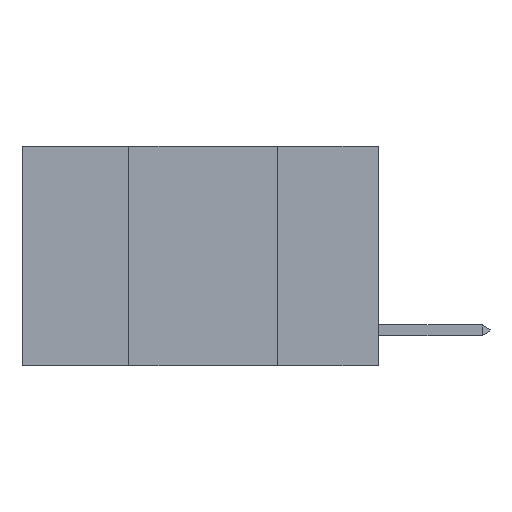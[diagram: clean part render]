
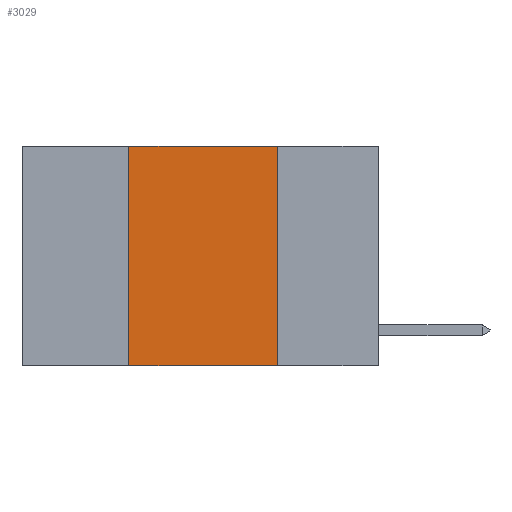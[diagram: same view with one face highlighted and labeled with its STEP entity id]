
A CAD part, left-side view. The second image highlights one B-rep face of the part: STEP entity #3029.
In plain terms, the highlighted planar face has unit normal (-1, 0, 0).
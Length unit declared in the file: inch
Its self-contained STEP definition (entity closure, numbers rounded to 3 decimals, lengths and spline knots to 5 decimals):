
#26 = LINE ( 'NONE', #12752, #2441 ) ;
#378 = EDGE_LOOP ( 'NONE', ( #12110, #11061, #12465, #7243 ) ) ;
#588 = VERTEX_POINT ( 'NONE', #13567 ) ;
#747 = EDGE_CURVE ( 'NONE', #1272, #11423, #3731, .T. ) ;
#1272 = VERTEX_POINT ( 'NONE', #5514 ) ;
#2012 = CARTESIAN_POINT ( 'NONE',  ( 0., 0.17, 0. ) ) ;
#2441 = VECTOR ( 'NONE', #4558, 39.37008 ) ;
#3029 = ADVANCED_FACE ( 'NONE', ( #9749 ), #10938, .F. ) ;
#3731 = LINE ( 'NONE', #7173, #7349 ) ;
#3758 = CARTESIAN_POINT ( 'NONE',  ( 0., 0.6, 0. ) ) ;
#3808 = DIRECTION ( 'NONE',  ( 1., 0., 0. ) ) ;
#4335 = CARTESIAN_POINT ( 'NONE',  ( 0., 0.42, 0. ) ) ;
#4558 = DIRECTION ( 'NONE',  ( 0., 0., -1. ) ) ;
#4739 = AXIS2_PLACEMENT_3D ( 'NONE', #3758, #3808, #12053 ) ;
#5514 = CARTESIAN_POINT ( 'NONE',  ( 0., 0.42, 0. ) ) ;
#5657 = VECTOR ( 'NONE', #12239, 39.37008 ) ;
#7173 = CARTESIAN_POINT ( 'NONE',  ( 0., 0.6, 0. ) ) ;
#7243 = ORIENTED_EDGE ( 'NONE', *, *, #7673, .T. ) ;
#7298 = DIRECTION ( 'NONE',  ( 0., -1., 0. ) ) ;
#7349 = VECTOR ( 'NONE', #7298, 39.37008 ) ;
#7673 = EDGE_CURVE ( 'NONE', #588, #11978, #9214, .T. ) ;
#8471 = EDGE_CURVE ( 'NONE', #588, #1272, #12982, .T. ) ;
#8855 = CARTESIAN_POINT ( 'NONE',  ( 0., 0.17, -0.37 ) ) ;
#9214 = LINE ( 'NONE', #11125, #5657 ) ;
#9749 = FACE_OUTER_BOUND ( 'NONE', #378, .T. ) ;
#10035 = EDGE_CURVE ( 'NONE', #11423, #11978, #26, .T. ) ;
#10938 = PLANE ( 'NONE',  #4739 ) ;
#11061 = ORIENTED_EDGE ( 'NONE', *, *, #747, .F. ) ;
#11125 = CARTESIAN_POINT ( 'NONE',  ( 0., 0.6, -0.37 ) ) ;
#11423 = VERTEX_POINT ( 'NONE', #2012 ) ;
#11978 = VERTEX_POINT ( 'NONE', #8855 ) ;
#12053 = DIRECTION ( 'NONE',  ( 0., 0., -1. ) ) ;
#12110 = ORIENTED_EDGE ( 'NONE', *, *, #10035, .F. ) ;
#12239 = DIRECTION ( 'NONE',  ( 0., -1., 0. ) ) ;
#12465 = ORIENTED_EDGE ( 'NONE', *, *, #8471, .F. ) ;
#12544 = DIRECTION ( 'NONE',  ( 0., 0., 1. ) ) ;
#12752 = CARTESIAN_POINT ( 'NONE',  ( 0., 0.17, 0. ) ) ;
#12982 = LINE ( 'NONE', #4335, #13314 ) ;
#13314 = VECTOR ( 'NONE', #12544, 39.37008 ) ;
#13567 = CARTESIAN_POINT ( 'NONE',  ( 0., 0.42, -0.37 ) ) ;
